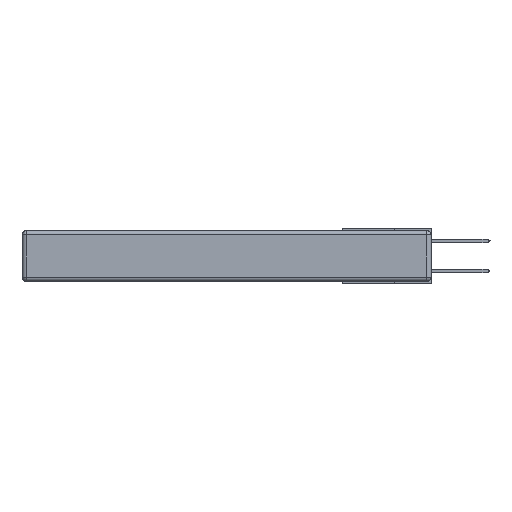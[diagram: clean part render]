
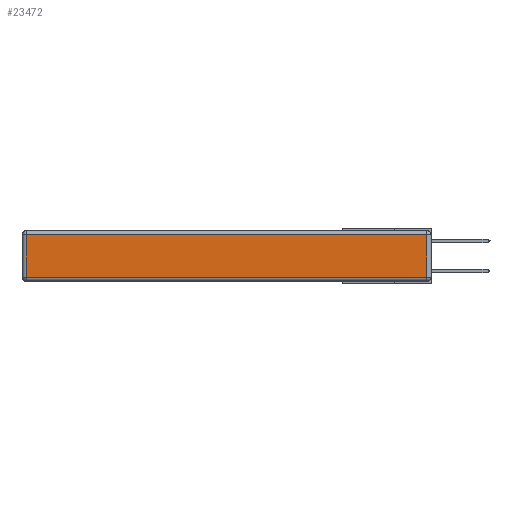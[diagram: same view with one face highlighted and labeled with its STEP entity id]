
A CAD part, left-side view. The second image highlights one B-rep face of the part: STEP entity #23472.
In plain terms, the highlighted planar face has unit normal (-1, 0, 0).
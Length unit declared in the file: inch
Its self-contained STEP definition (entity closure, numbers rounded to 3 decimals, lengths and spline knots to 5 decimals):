
#471 = CARTESIAN_POINT ( 'NONE',  ( 0., 0.03, -0.03 ) ) ;
#2174 = CARTESIAN_POINT ( 'NONE',  ( 0., 2.72, -0.313 ) ) ;
#3522 = CARTESIAN_POINT ( 'NONE',  ( 0., 2.75, -0.03 ) ) ;
#3978 = CARTESIAN_POINT ( 'NONE',  ( 0., 0., -0.313 ) ) ;
#4094 = CARTESIAN_POINT ( 'NONE',  ( 0., 0., -0.343 ) ) ;
#4108 = EDGE_LOOP ( 'NONE', ( #24611, #4387, #6735, #8620 ) ) ;
#4387 = ORIENTED_EDGE ( 'NONE', *, *, #10398, .T. ) ;
#5896 = DIRECTION ( 'NONE',  ( 0., -1., 0. ) ) ;
#6735 = ORIENTED_EDGE ( 'NONE', *, *, #17091, .T. ) ;
#7509 = VECTOR ( 'NONE', #17308, 39.37008 ) ;
#7711 = VERTEX_POINT ( 'NONE', #2174 ) ;
#8092 = DIRECTION ( 'NONE',  ( 0., 0., 1. ) ) ;
#8620 = ORIENTED_EDGE ( 'NONE', *, *, #10450, .T. ) ;
#8999 = CARTESIAN_POINT ( 'NONE',  ( 0., 2.72, -0.343 ) ) ;
#10398 = EDGE_CURVE ( 'NONE', #22636, #18106, #12138, .T. ) ;
#10450 = EDGE_CURVE ( 'NONE', #25479, #7711, #13100, .T. ) ;
#10600 = PLANE ( 'NONE',  #23498 ) ;
#12138 = LINE ( 'NONE', #21389, #23155 ) ;
#12337 = DIRECTION ( 'NONE',  ( -1., 0., 0. ) ) ;
#13100 = LINE ( 'NONE', #8999, #7509 ) ;
#14285 = LINE ( 'NONE', #3978, #19808 ) ;
#15316 = DIRECTION ( 'NONE',  ( 0., 0., 1. ) ) ;
#16956 = VECTOR ( 'NONE', #22022, 39.37008 ) ;
#17091 = EDGE_CURVE ( 'NONE', #18106, #25479, #18527, .T. ) ;
#17308 = DIRECTION ( 'NONE',  ( 0., 0., -1. ) ) ;
#18106 = VERTEX_POINT ( 'NONE', #471 ) ;
#18527 = LINE ( 'NONE', #3522, #16956 ) ;
#19808 = VECTOR ( 'NONE', #5896, 39.37008 ) ;
#21389 = CARTESIAN_POINT ( 'NONE',  ( 0., 0.03, -0.343 ) ) ;
#21596 = FACE_OUTER_BOUND ( 'NONE', #4108, .T. ) ;
#22022 = DIRECTION ( 'NONE',  ( 0., 1., 0. ) ) ;
#22425 = CARTESIAN_POINT ( 'NONE',  ( 0., 0.03, -0.313 ) ) ;
#22636 = VERTEX_POINT ( 'NONE', #22425 ) ;
#23155 = VECTOR ( 'NONE', #15316, 39.37008 ) ;
#23472 = ADVANCED_FACE ( 'NONE', ( #21596 ), #10600, .T. ) ;
#23498 = AXIS2_PLACEMENT_3D ( 'NONE', #4094, #12337, #8092 ) ;
#24611 = ORIENTED_EDGE ( 'NONE', *, *, #24779, .T. ) ;
#24779 = EDGE_CURVE ( 'NONE', #7711, #22636, #14285, .T. ) ;
#25362 = CARTESIAN_POINT ( 'NONE',  ( 0., 2.72, -0.03 ) ) ;
#25479 = VERTEX_POINT ( 'NONE', #25362 ) ;
